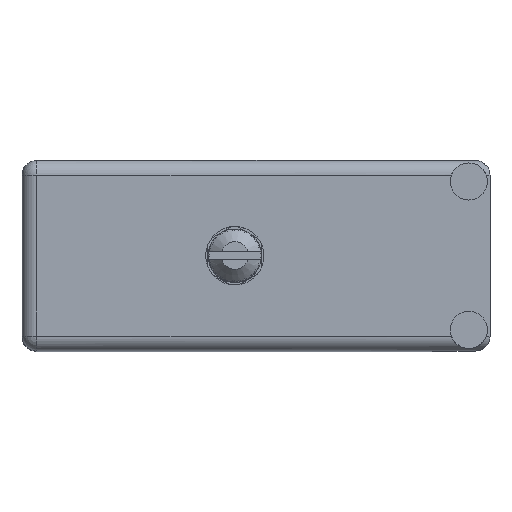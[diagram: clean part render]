
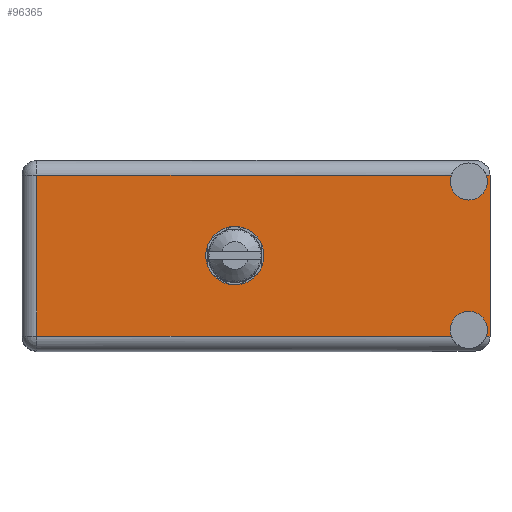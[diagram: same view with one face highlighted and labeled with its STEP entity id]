
A CAD part, top view. The second image highlights one B-rep face of the part: STEP entity #96365.
In plain terms, the highlighted face is planar.
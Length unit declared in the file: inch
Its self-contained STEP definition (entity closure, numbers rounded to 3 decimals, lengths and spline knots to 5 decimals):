
#2657 = CARTESIAN_POINT ( 'NONE',  ( 2.108, 1.566, -0.0995 ) ) ;
#2853 = CIRCLE ( 'NONE', #47199, 0.0875 ) ;
#3115 = VERTEX_POINT ( 'NONE', #58028 ) ;
#4028 = ORIENTED_EDGE ( 'NONE', *, *, #66168, .F. ) ;
#5649 = CARTESIAN_POINT ( 'NONE',  ( 0., 1.566, -0.899 ) ) ;
#6785 = CARTESIAN_POINT ( 'NONE',  ( 0., 1.566, -0.829 ) ) ;
#7983 = DIRECTION ( 'NONE',  ( 1., 0., 0. ) ) ;
#9388 = AXIS2_PLACEMENT_3D ( 'NONE', #67613, #14677, #84460 ) ;
#9850 = ORIENTED_EDGE ( 'NONE', *, *, #101688, .T. ) ;
#10409 = CARTESIAN_POINT ( 'NONE',  ( 2.108, 1.566, -0.7995 ) ) ;
#11259 = EDGE_CURVE ( 'NONE', #32504, #35763, #107092, .T. ) ;
#12209 = CARTESIAN_POINT ( 'NONE',  ( 2.208, 1.566, -0.07 ) ) ;
#12272 = VERTEX_POINT ( 'NONE', #45519 ) ;
#14677 = DIRECTION ( 'NONE',  ( 0., 1., 0. ) ) ;
#15168 = ORIENTED_EDGE ( 'NONE', *, *, #55177, .F. ) ;
#15229 = DIRECTION ( 'NONE',  ( -1., 0., 0. ) ) ;
#17254 = CARTESIAN_POINT ( 'NONE',  ( 2.19038, 1.566, -0.07 ) ) ;
#19366 = VERTEX_POINT ( 'NONE', #110905 ) ;
#19958 = VERTEX_POINT ( 'NONE', #60402 ) ;
#20805 = DIRECTION ( 'NONE',  ( -1., 0., 0. ) ) ;
#21082 = CIRCLE ( 'NONE', #109539, 0.0875 ) ;
#21812 = VECTOR ( 'NONE', #60386, 39.37008 ) ;
#23149 = EDGE_CURVE ( 'NONE', #58685, #29734, #21082, .T. ) ;
#24915 = DIRECTION ( 'NONE',  ( 0., 0., 1. ) ) ;
#25579 = EDGE_LOOP ( 'NONE', ( #37424, #39923 ) ) ;
#25902 = LINE ( 'NONE', #72453, #67106 ) ;
#25936 = VERTEX_POINT ( 'NONE', #88078 ) ;
#27617 = EDGE_CURVE ( 'NONE', #3115, #40675, #87642, .T. ) ;
#27673 = CARTESIAN_POINT ( 'NONE',  ( 2.108, 1.566, -0.7995 ) ) ;
#27969 = DIRECTION ( 'NONE',  ( 0., 1., 0. ) ) ;
#28373 = DIRECTION ( 'NONE',  ( 0., 0., 1. ) ) ;
#29092 = CARTESIAN_POINT ( 'NONE',  ( 1.004, 1.566, -0.4495 ) ) ;
#29734 = VERTEX_POINT ( 'NONE', #91644 ) ;
#30948 = LINE ( 'NONE', #6785, #103707 ) ;
#31374 = DIRECTION ( 'NONE',  ( 0., 1., 0. ) ) ;
#31607 = EDGE_LOOP ( 'NONE', ( #42806, #101468, #110119, #41693, #4028, #9850, #15168, #34083, #37877, #112113 ) ) ;
#32504 = VERTEX_POINT ( 'NONE', #17254 ) ;
#34083 = ORIENTED_EDGE ( 'NONE', *, *, #27617, .F. ) ;
#35763 = VERTEX_POINT ( 'NONE', #97202 ) ;
#37424 = ORIENTED_EDGE ( 'NONE', *, *, #99527, .F. ) ;
#37877 = ORIENTED_EDGE ( 'NONE', *, *, #84452, .T. ) ;
#39031 = DIRECTION ( 'NONE',  ( 0., 0., 1. ) ) ;
#39923 = ORIENTED_EDGE ( 'NONE', *, *, #43150, .F. ) ;
#40675 = VERTEX_POINT ( 'NONE', #110789 ) ;
#41693 = ORIENTED_EDGE ( 'NONE', *, *, #11259, .T. ) ;
#42806 = ORIENTED_EDGE ( 'NONE', *, *, #48813, .T. ) ;
#43150 = EDGE_CURVE ( 'NONE', #67935, #86702, #103407, .T. ) ;
#43470 = DIRECTION ( 'NONE',  ( 0., 1., 0. ) ) ;
#43613 = VECTOR ( 'NONE', #20805, 39.37008 ) ;
#43862 = LINE ( 'NONE', #51519, #21812 ) ;
#45016 = FACE_OUTER_BOUND ( 'NONE', #31607, .T. ) ;
#45519 = CARTESIAN_POINT ( 'NONE',  ( 2.208, 1.566, -0.829 ) ) ;
#47199 = AXIS2_PLACEMENT_3D ( 'NONE', #10409, #80613, #28373 ) ;
#48813 = EDGE_CURVE ( 'NONE', #25936, #29734, #57475, .T. ) ;
#49248 = VECTOR ( 'NONE', #65473, 39.37008 ) ;
#49330 = EDGE_CURVE ( 'NONE', #19958, #25936, #43862, .T. ) ;
#51204 = CARTESIAN_POINT ( 'NONE',  ( 1.004, 1.566, -0.587 ) ) ;
#51519 = CARTESIAN_POINT ( 'NONE',  ( 0.07, 1.566, -0.899 ) ) ;
#55177 = EDGE_CURVE ( 'NONE', #40675, #19366, #2853, .T. ) ;
#57169 = AXIS2_PLACEMENT_3D ( 'NONE', #27673, #43470, #70313 ) ;
#57475 = LINE ( 'NONE', #12209, #49248 ) ;
#58028 = CARTESIAN_POINT ( 'NONE',  ( 2.02562, 1.566, -0.829 ) ) ;
#58601 = EDGE_CURVE ( 'NONE', #32504, #58685, #86924, .T. ) ;
#58685 = VERTEX_POINT ( 'NONE', #92315 ) ;
#59343 = AXIS2_PLACEMENT_3D ( 'NONE', #2657, #27969, #98917 ) ;
#59864 = CARTESIAN_POINT ( 'NONE',  ( 2.108, 1.566, -0.0995 ) ) ;
#60386 = DIRECTION ( 'NONE',  ( 0., 0., 1. ) ) ;
#60402 = CARTESIAN_POINT ( 'NONE',  ( 0.07, 1.566, -0.829 ) ) ;
#64151 = LINE ( 'NONE', #97496, #43613 ) ;
#65473 = DIRECTION ( 'NONE',  ( 1., 0., 0. ) ) ;
#66168 = EDGE_CURVE ( 'NONE', #12272, #35763, #25902, .T. ) ;
#67106 = VECTOR ( 'NONE', #39031, 39.37008 ) ;
#67613 = CARTESIAN_POINT ( 'NONE',  ( 1.004, 1.566, -0.4495 ) ) ;
#67935 = VERTEX_POINT ( 'NONE', #51204 ) ;
#68995 = CARTESIAN_POINT ( 'NONE',  ( 2.208, 1.566, -0.07 ) ) ;
#70313 = DIRECTION ( 'NONE',  ( 0., 0., 1. ) ) ;
#72453 = CARTESIAN_POINT ( 'NONE',  ( 2.208, 1.566, 0. ) ) ;
#73648 = DIRECTION ( 'NONE',  ( 0., 1., 0. ) ) ;
#74270 = VECTOR ( 'NONE', #7983, 39.37008 ) ;
#77526 = DIRECTION ( 'NONE',  ( 0., 1., 0. ) ) ;
#79675 = AXIS2_PLACEMENT_3D ( 'NONE', #5649, #31374, #110278 ) ;
#80247 = CIRCLE ( 'NONE', #9388, 0.1375 ) ;
#80613 = DIRECTION ( 'NONE',  ( 0., 1., 0. ) ) ;
#80698 = FACE_BOUND ( 'NONE', #25579, .T. ) ;
#81752 = AXIS2_PLACEMENT_3D ( 'NONE', #29092, #73648, #108446 ) ;
#83933 = PLANE ( 'NONE',  #79675 ) ;
#84452 = EDGE_CURVE ( 'NONE', #3115, #19958, #64151, .T. ) ;
#84460 = DIRECTION ( 'NONE',  ( 0., 0., 1. ) ) ;
#86702 = VERTEX_POINT ( 'NONE', #96373 ) ;
#86924 = CIRCLE ( 'NONE', #59343, 0.0875 ) ;
#87642 = CIRCLE ( 'NONE', #57169, 0.0875 ) ;
#88078 = CARTESIAN_POINT ( 'NONE',  ( 0.07, 1.566, -0.07 ) ) ;
#91644 = CARTESIAN_POINT ( 'NONE',  ( 2.02562, 1.566, -0.07 ) ) ;
#92315 = CARTESIAN_POINT ( 'NONE',  ( 2.108, 1.566, -0.187 ) ) ;
#96365 = ADVANCED_FACE ( 'NONE', ( #80698, #45016 ), #83933, .T. ) ;
#96373 = CARTESIAN_POINT ( 'NONE',  ( 1.004, 1.566, -0.312 ) ) ;
#97202 = CARTESIAN_POINT ( 'NONE',  ( 2.208, 1.566, -0.07 ) ) ;
#97496 = CARTESIAN_POINT ( 'NONE',  ( 0., 1.566, -0.829 ) ) ;
#98917 = DIRECTION ( 'NONE',  ( 0., 0., 1. ) ) ;
#99527 = EDGE_CURVE ( 'NONE', #86702, #67935, #80247, .T. ) ;
#101468 = ORIENTED_EDGE ( 'NONE', *, *, #23149, .F. ) ;
#101688 = EDGE_CURVE ( 'NONE', #12272, #19366, #30948, .T. ) ;
#103407 = CIRCLE ( 'NONE', #81752, 0.1375 ) ;
#103707 = VECTOR ( 'NONE', #15229, 39.37008 ) ;
#107092 = LINE ( 'NONE', #68995, #74270 ) ;
#108446 = DIRECTION ( 'NONE',  ( 0., 0., 1. ) ) ;
#109539 = AXIS2_PLACEMENT_3D ( 'NONE', #59864, #77526, #24915 ) ;
#110119 = ORIENTED_EDGE ( 'NONE', *, *, #58601, .F. ) ;
#110278 = DIRECTION ( 'NONE',  ( 0., 0., 1. ) ) ;
#110789 = CARTESIAN_POINT ( 'NONE',  ( 2.108, 1.566, -0.712 ) ) ;
#110905 = CARTESIAN_POINT ( 'NONE',  ( 2.19038, 1.566, -0.829 ) ) ;
#112113 = ORIENTED_EDGE ( 'NONE', *, *, #49330, .T. ) ;
